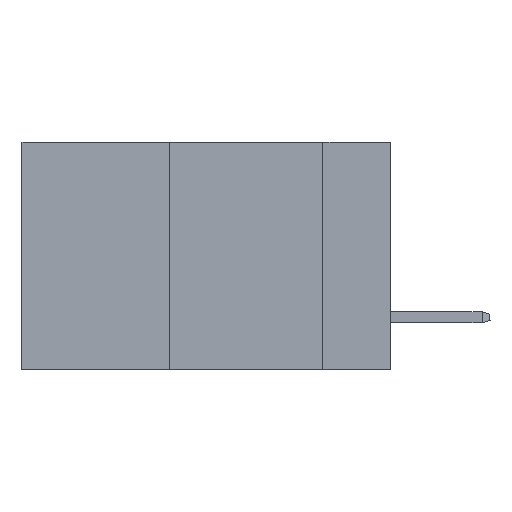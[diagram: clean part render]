
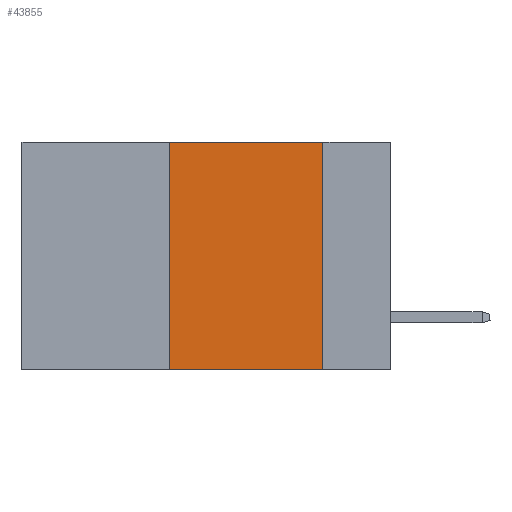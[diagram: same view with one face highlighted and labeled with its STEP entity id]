
A CAD part, left-side view. The second image highlights one B-rep face of the part: STEP entity #43855.
In plain terms, the highlighted planar face has unit normal (-1, 0, 0).
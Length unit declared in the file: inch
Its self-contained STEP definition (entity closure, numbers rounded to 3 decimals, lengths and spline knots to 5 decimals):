
#1284 = CARTESIAN_POINT ( 'NONE',  ( 0., 0.36, 0. ) ) ;
#1443 = DIRECTION ( 'NONE',  ( 1., 0., 0. ) ) ;
#1678 = DIRECTION ( 'NONE',  ( 0., -1., 0. ) ) ;
#7730 = VERTEX_POINT ( 'NONE', #28575 ) ;
#7984 = VECTOR ( 'NONE', #37436, 39.37008 ) ;
#8372 = ORIENTED_EDGE ( 'NONE', *, *, #34769, .F. ) ;
#9179 = LINE ( 'NONE', #12767, #7984 ) ;
#10312 = EDGE_CURVE ( 'NONE', #40617, #36906, #16715, .T. ) ;
#10627 = VERTEX_POINT ( 'NONE', #1284 ) ;
#12767 = CARTESIAN_POINT ( 'NONE',  ( 0., 0.6, -0.37 ) ) ;
#13491 = DIRECTION ( 'NONE',  ( 0., 0., -1. ) ) ;
#14963 = ORIENTED_EDGE ( 'NONE', *, *, #10312, .F. ) ;
#15915 = EDGE_CURVE ( 'NONE', #7730, #10627, #44348, .T. ) ;
#16715 = LINE ( 'NONE', #32094, #35582 ) ;
#18181 = FACE_OUTER_BOUND ( 'NONE', #27051, .T. ) ;
#19435 = AXIS2_PLACEMENT_3D ( 'NONE', #19749, #1443, #34816 ) ;
#19749 = CARTESIAN_POINT ( 'NONE',  ( 0., 0.6, 0. ) ) ;
#19911 = PLANE ( 'NONE',  #19435 ) ;
#20782 = ORIENTED_EDGE ( 'NONE', *, *, #27880, .T. ) ;
#22996 = CARTESIAN_POINT ( 'NONE',  ( 0., 0.6, 0. ) ) ;
#25617 = VECTOR ( 'NONE', #1678, 39.37008 ) ;
#27051 = EDGE_LOOP ( 'NONE', ( #14963, #8372, #39719, #20782 ) ) ;
#27880 = EDGE_CURVE ( 'NONE', #7730, #36906, #9179, .T. ) ;
#28169 = CARTESIAN_POINT ( 'NONE',  ( 0., 0.11, 0. ) ) ;
#28575 = CARTESIAN_POINT ( 'NONE',  ( 0., 0.36, -0.37 ) ) ;
#31016 = VECTOR ( 'NONE', #47897, 39.37008 ) ;
#32094 = CARTESIAN_POINT ( 'NONE',  ( 0., 0.11, 0. ) ) ;
#34769 = EDGE_CURVE ( 'NONE', #10627, #40617, #47631, .T. ) ;
#34816 = DIRECTION ( 'NONE',  ( 0., 0., -1. ) ) ;
#35582 = VECTOR ( 'NONE', #13491, 39.37008 ) ;
#36906 = VERTEX_POINT ( 'NONE', #43539 ) ;
#37436 = DIRECTION ( 'NONE',  ( 0., -1., 0. ) ) ;
#39719 = ORIENTED_EDGE ( 'NONE', *, *, #15915, .F. ) ;
#40617 = VERTEX_POINT ( 'NONE', #28169 ) ;
#43539 = CARTESIAN_POINT ( 'NONE',  ( 0., 0.11, -0.37 ) ) ;
#43855 = ADVANCED_FACE ( 'NONE', ( #18181 ), #19911, .F. ) ;
#44348 = LINE ( 'NONE', #47424, #31016 ) ;
#47424 = CARTESIAN_POINT ( 'NONE',  ( 0., 0.36, 0. ) ) ;
#47631 = LINE ( 'NONE', #22996, #25617 ) ;
#47897 = DIRECTION ( 'NONE',  ( 0., 0., 1. ) ) ;
